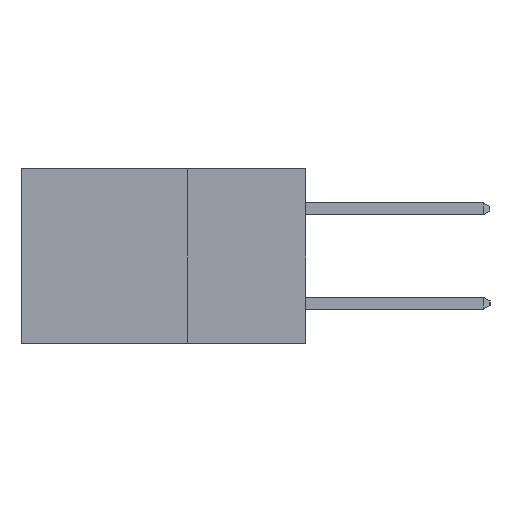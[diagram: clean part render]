
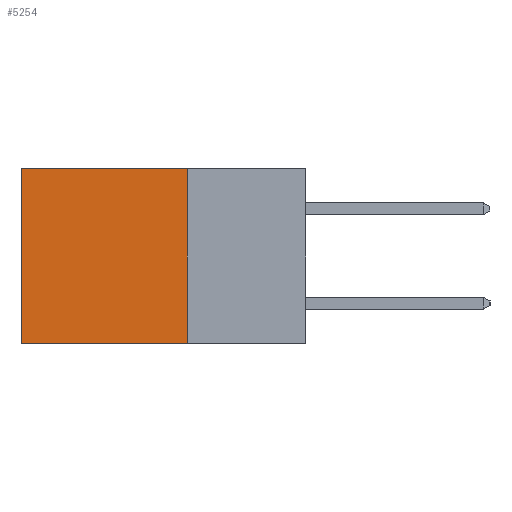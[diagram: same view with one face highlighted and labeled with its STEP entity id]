
A CAD part, left-side view. The second image highlights one B-rep face of the part: STEP entity #5254.
In plain terms, the highlighted planar face has unit normal (-1, 0, 0).
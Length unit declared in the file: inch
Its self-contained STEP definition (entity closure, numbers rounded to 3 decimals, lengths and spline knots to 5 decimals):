
#684 = DIRECTION ( 'NONE',  ( 0., 1., 0. ) ) ;
#969 = VERTEX_POINT ( 'NONE', #1768 ) ;
#992 = VECTOR ( 'NONE', #4050, 39.37008 ) ;
#1089 = ORIENTED_EDGE ( 'NONE', *, *, #7991, .F. ) ;
#1664 = ORIENTED_EDGE ( 'NONE', *, *, #8569, .T. ) ;
#1731 = CARTESIAN_POINT ( 'NONE',  ( 0.2615, 0.6, -0.37 ) ) ;
#1768 = CARTESIAN_POINT ( 'NONE',  ( 0.2615, 0.6, 0. ) ) ;
#2890 = CARTESIAN_POINT ( 'NONE',  ( 0.2615, 0.25, -0.37 ) ) ;
#2915 = CARTESIAN_POINT ( 'NONE',  ( 0.2615, 0.25, 0. ) ) ;
#3158 = VECTOR ( 'NONE', #684, 39.37008 ) ;
#3423 = CARTESIAN_POINT ( 'NONE',  ( 0.2615, 0.6, -0.37 ) ) ;
#4050 = DIRECTION ( 'NONE',  ( 0., 0., -1. ) ) ;
#5254 = ADVANCED_FACE ( 'NONE', ( #7377 ), #6211, .F. ) ;
#5649 = DIRECTION ( 'NONE',  ( 0., 1., 0. ) ) ;
#5674 = DIRECTION ( 'NONE',  ( 0., 0., -1. ) ) ;
#5844 = CARTESIAN_POINT ( 'NONE',  ( 0.2615, 0.25, -0.37 ) ) ;
#6158 = DIRECTION ( 'NONE',  ( 0., 0., -1. ) ) ;
#6163 = DIRECTION ( 'NONE',  ( 1., 0., 0. ) ) ;
#6189 = CARTESIAN_POINT ( 'NONE',  ( 0.2615, 0.25, -0.37 ) ) ;
#6211 = PLANE ( 'NONE',  #15742 ) ;
#6336 = EDGE_CURVE ( 'NONE', #15570, #16289, #10309, .T. ) ;
#6805 = EDGE_CURVE ( 'NONE', #969, #16289, #11351, .T. ) ;
#7055 = LINE ( 'NONE', #5844, #10655 ) ;
#7377 = FACE_OUTER_BOUND ( 'NONE', #17217, .T. ) ;
#7991 = EDGE_CURVE ( 'NONE', #8277, #15570, #7055, .T. ) ;
#8277 = VERTEX_POINT ( 'NONE', #2915 ) ;
#8307 = CARTESIAN_POINT ( 'NONE',  ( 0.2615, 0.25, -0.37 ) ) ;
#8569 = EDGE_CURVE ( 'NONE', #8277, #969, #9349, .T. ) ;
#9349 = LINE ( 'NONE', #12338, #12138 ) ;
#10309 = LINE ( 'NONE', #2890, #3158 ) ;
#10655 = VECTOR ( 'NONE', #5674, 39.37008 ) ;
#11351 = LINE ( 'NONE', #3423, #992 ) ;
#12138 = VECTOR ( 'NONE', #5649, 39.37008 ) ;
#12338 = CARTESIAN_POINT ( 'NONE',  ( 0.2615, 0.25, 0. ) ) ;
#12591 = ORIENTED_EDGE ( 'NONE', *, *, #6336, .F. ) ;
#15570 = VERTEX_POINT ( 'NONE', #8307 ) ;
#15742 = AXIS2_PLACEMENT_3D ( 'NONE', #6189, #6163, #6158 ) ;
#16289 = VERTEX_POINT ( 'NONE', #1731 ) ;
#16975 = ORIENTED_EDGE ( 'NONE', *, *, #6805, .T. ) ;
#17217 = EDGE_LOOP ( 'NONE', ( #16975, #12591, #1089, #1664 ) ) ;
